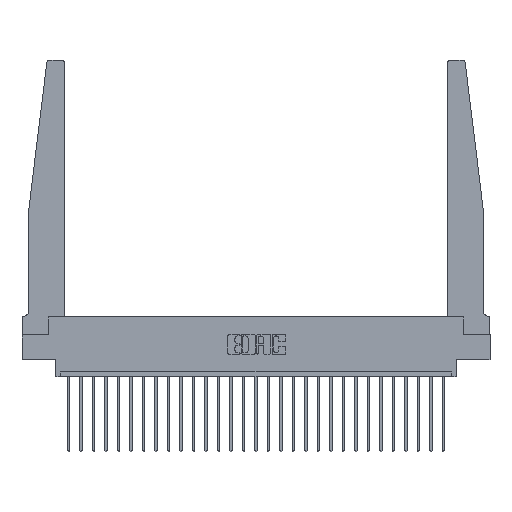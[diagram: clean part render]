
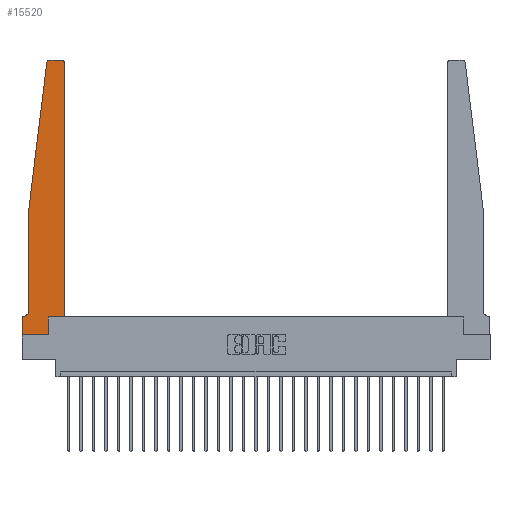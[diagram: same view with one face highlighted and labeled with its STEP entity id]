
A CAD part, top view. The second image highlights one B-rep face of the part: STEP entity #15520.
In plain terms, the highlighted planar face has unit normal (0, 0, 1).
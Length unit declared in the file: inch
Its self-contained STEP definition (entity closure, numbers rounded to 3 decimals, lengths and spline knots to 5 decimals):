
#134 = DIRECTION ( 'NONE',  ( 0., -1., 0. ) ) ;
#464 = VECTOR ( 'NONE', #134, 39.37008 ) ;
#761 = CARTESIAN_POINT ( 'NONE',  ( 0.425, 0.18, 0.37 ) ) ;
#1050 = EDGE_CURVE ( 'NONE', #2576, #16049, #16598, .T. ) ;
#1528 = EDGE_CURVE ( 'NONE', #13641, #16543, #20681, .T. ) ;
#2321 = VECTOR ( 'NONE', #21453, 39.37008 ) ;
#2568 = DIRECTION ( 'NONE',  ( 0., 0., 1. ) ) ;
#2576 = VERTEX_POINT ( 'NONE', #4182 ) ;
#2856 = LINE ( 'NONE', #14969, #464 ) ;
#2903 = DIRECTION ( 'NONE',  ( 1., 0., 0. ) ) ;
#3430 = DIRECTION ( 'NONE',  ( -1., 0., 0. ) ) ;
#3641 = CARTESIAN_POINT ( 'NONE',  ( 0.2605, 0.18, 0.37 ) ) ;
#3824 = VECTOR ( 'NONE', #11043, 39.37008 ) ;
#4100 = EDGE_CURVE ( 'NONE', #11266, #21695, #5298, .T. ) ;
#4182 = CARTESIAN_POINT ( 'NONE',  ( 0.395, 2.75, 0.37 ) ) ;
#4590 = AXIS2_PLACEMENT_3D ( 'NONE', #21579, #19865, #15497 ) ;
#4611 = CARTESIAN_POINT ( 'NONE',  ( 0.015, 0.1875, 0.37 ) ) ;
#4756 = CARTESIAN_POINT ( 'NONE',  ( 0., 0.1875, 0.37 ) ) ;
#5124 = CARTESIAN_POINT ( 'NONE',  ( 0.425, 2.72, 0.37 ) ) ;
#5199 = DIRECTION ( 'NONE',  ( 0., 0., -1. ) ) ;
#5298 = LINE ( 'NONE', #8982, #22203 ) ;
#5752 = VERTEX_POINT ( 'NONE', #4756 ) ;
#5806 = EDGE_CURVE ( 'NONE', #8053, #5752, #21113, .T. ) ;
#5840 = CARTESIAN_POINT ( 'NONE',  ( 0.065, 0.2375, 0.37 ) ) ;
#5869 = ORIENTED_EDGE ( 'NONE', *, *, #14601, .T. ) ;
#6216 = VECTOR ( 'NONE', #18634, 39.37008 ) ;
#6264 = ORIENTED_EDGE ( 'NONE', *, *, #1050, .T. ) ;
#6447 = CARTESIAN_POINT ( 'NONE',  ( 0.25, 2.75, 0.37 ) ) ;
#6609 = LINE ( 'NONE', #14131, #6216 ) ;
#6911 = ORIENTED_EDGE ( 'NONE', *, *, #23946, .T. ) ;
#7809 = ORIENTED_EDGE ( 'NONE', *, *, #13387, .T. ) ;
#7904 = VECTOR ( 'NONE', #3430, 39.37008 ) ;
#8053 = VERTEX_POINT ( 'NONE', #4611 ) ;
#8982 = CARTESIAN_POINT ( 'NONE',  ( 0.065, 1.25, 0.37 ) ) ;
#9003 = DIRECTION ( 'NONE',  ( -1., 0., 0. ) ) ;
#9606 = CARTESIAN_POINT ( 'NONE',  ( 0.065, 0.1875, 0.37 ) ) ;
#9836 = AXIS2_PLACEMENT_3D ( 'NONE', #24668, #22672, #2903 ) ;
#9869 = EDGE_CURVE ( 'NONE', #23331, #2576, #20183, .T. ) ;
#10279 = VERTEX_POINT ( 'NONE', #17724 ) ;
#11043 = DIRECTION ( 'NONE',  ( 1., 0., 0. ) ) ;
#11266 = VERTEX_POINT ( 'NONE', #20382 ) ;
#11473 = ORIENTED_EDGE ( 'NONE', *, *, #5806, .T. ) ;
#12477 = DIRECTION ( 'NONE',  ( 1., 0., 0. ) ) ;
#13010 = CARTESIAN_POINT ( 'NONE',  ( 0.27653, 2.75, 0.37 ) ) ;
#13023 = LINE ( 'NONE', #21593, #3824 ) ;
#13248 = DIRECTION ( 'NONE',  ( -0.122, -0.992, 0. ) ) ;
#13372 = LINE ( 'NONE', #25405, #22349 ) ;
#13387 = EDGE_CURVE ( 'NONE', #10279, #19941, #13023, .T. ) ;
#13437 = AXIS2_PLACEMENT_3D ( 'NONE', #24590, #2568, #16530 ) ;
#13523 = LINE ( 'NONE', #3641, #2321 ) ;
#13641 = VERTEX_POINT ( 'NONE', #24360 ) ;
#14131 = CARTESIAN_POINT ( 'NONE',  ( 0.425, 0.18, 0.37 ) ) ;
#14601 = EDGE_CURVE ( 'NONE', #21695, #8053, #17006, .T. ) ;
#14969 = CARTESIAN_POINT ( 'NONE',  ( 0., 0., 0.37 ) ) ;
#15445 = CARTESIAN_POINT ( 'NONE',  ( 0.24675, 2.72367, 0.37 ) ) ;
#15497 = DIRECTION ( 'NONE',  ( 1., 0., 0. ) ) ;
#15520 = ADVANCED_FACE ( 'NONE', ( #20959 ), #16602, .T. ) ;
#16049 = VERTEX_POINT ( 'NONE', #13010 ) ;
#16125 = ORIENTED_EDGE ( 'NONE', *, *, #24744, .T. ) ;
#16381 = EDGE_LOOP ( 'NONE', ( #6264, #6911, #24888, #19456, #5869, #11473, #16125, #7809, #21811, #21533, #24591, #20040 ) ) ;
#16485 = CARTESIAN_POINT ( 'NONE',  ( 0.425, 0.18, 0.37 ) ) ;
#16530 = DIRECTION ( 'NONE',  ( 1., 0., 0. ) ) ;
#16543 = VERTEX_POINT ( 'NONE', #16485 ) ;
#16598 = LINE ( 'NONE', #6447, #23094 ) ;
#16602 = PLANE ( 'NONE',  #9836 ) ;
#17006 = CIRCLE ( 'NONE', #18715, 0.05 ) ;
#17109 = EDGE_CURVE ( 'NONE', #19941, #13641, #13523, .T. ) ;
#17161 = DIRECTION ( 'NONE',  ( 0., -1., 0. ) ) ;
#17724 = CARTESIAN_POINT ( 'NONE',  ( 0., 0., 0.37 ) ) ;
#18079 = VECTOR ( 'NONE', #12477, 39.37008 ) ;
#18095 = CIRCLE ( 'NONE', #13437, 0.03 ) ;
#18634 = DIRECTION ( 'NONE',  ( 0., 1., 0. ) ) ;
#18715 = AXIS2_PLACEMENT_3D ( 'NONE', #20773, #5199, #9003 ) ;
#19456 = ORIENTED_EDGE ( 'NONE', *, *, #4100, .T. ) ;
#19865 = DIRECTION ( 'NONE',  ( 0., 0., 1. ) ) ;
#19941 = VERTEX_POINT ( 'NONE', #23292 ) ;
#20040 = ORIENTED_EDGE ( 'NONE', *, *, #9869, .T. ) ;
#20183 = CIRCLE ( 'NONE', #4590, 0.03 ) ;
#20382 = CARTESIAN_POINT ( 'NONE',  ( 0.065, 1.25, 0.37 ) ) ;
#20681 = LINE ( 'NONE', #761, #18079 ) ;
#20708 = DIRECTION ( 'NONE',  ( -1., 0., 0. ) ) ;
#20773 = CARTESIAN_POINT ( 'NONE',  ( 0.015, 0.2375, 0.37 ) ) ;
#20959 = FACE_OUTER_BOUND ( 'NONE', #16381, .T. ) ;
#21113 = LINE ( 'NONE', #9606, #7904 ) ;
#21453 = DIRECTION ( 'NONE',  ( 0., 1., 0. ) ) ;
#21533 = ORIENTED_EDGE ( 'NONE', *, *, #1528, .T. ) ;
#21579 = CARTESIAN_POINT ( 'NONE',  ( 0.395, 2.72, 0.37 ) ) ;
#21593 = CARTESIAN_POINT ( 'NONE',  ( 0., 0., 0.37 ) ) ;
#21695 = VERTEX_POINT ( 'NONE', #5840 ) ;
#21808 = EDGE_CURVE ( 'NONE', #16543, #23331, #6609, .T. ) ;
#21811 = ORIENTED_EDGE ( 'NONE', *, *, #17109, .T. ) ;
#22203 = VECTOR ( 'NONE', #17161, 39.37008 ) ;
#22349 = VECTOR ( 'NONE', #13248, 39.37008 ) ;
#22672 = DIRECTION ( 'NONE',  ( 0., 0., 1. ) ) ;
#23094 = VECTOR ( 'NONE', #20708, 39.37008 ) ;
#23292 = CARTESIAN_POINT ( 'NONE',  ( 0.2605, 0., 0.37 ) ) ;
#23331 = VERTEX_POINT ( 'NONE', #5124 ) ;
#23946 = EDGE_CURVE ( 'NONE', #16049, #25413, #18095, .T. ) ;
#24360 = CARTESIAN_POINT ( 'NONE',  ( 0.2605, 0.18, 0.37 ) ) ;
#24590 = CARTESIAN_POINT ( 'NONE',  ( 0.27653, 2.72, 0.37 ) ) ;
#24591 = ORIENTED_EDGE ( 'NONE', *, *, #21808, .T. ) ;
#24668 = CARTESIAN_POINT ( 'NONE',  ( 0., 0.1875, 0.37 ) ) ;
#24744 = EDGE_CURVE ( 'NONE', #5752, #10279, #2856, .T. ) ;
#24853 = EDGE_CURVE ( 'NONE', #25413, #11266, #13372, .T. ) ;
#24888 = ORIENTED_EDGE ( 'NONE', *, *, #24853, .T. ) ;
#25405 = CARTESIAN_POINT ( 'NONE',  ( 0.065, 1.25, 0.37 ) ) ;
#25413 = VERTEX_POINT ( 'NONE', #15445 ) ;
